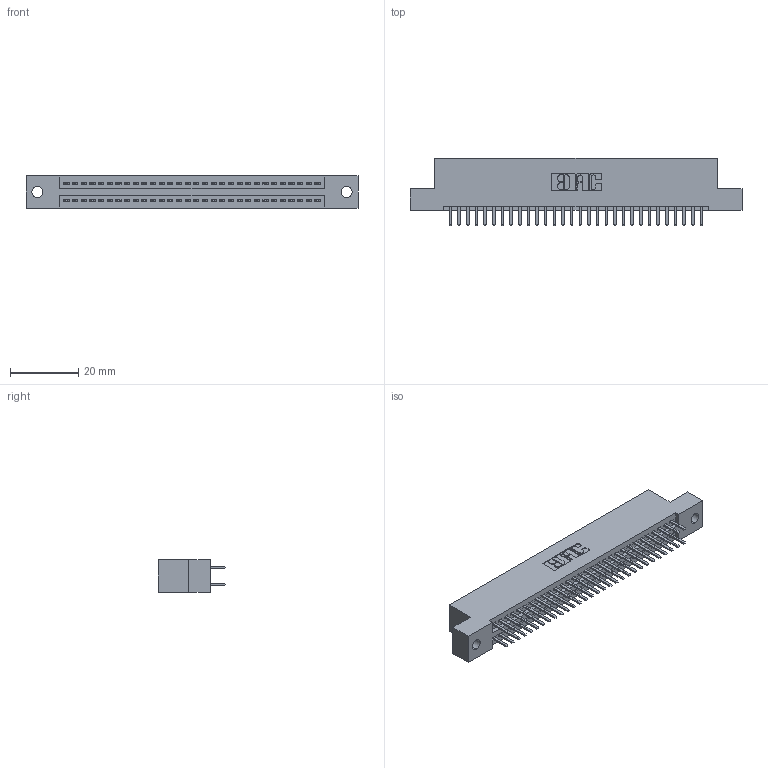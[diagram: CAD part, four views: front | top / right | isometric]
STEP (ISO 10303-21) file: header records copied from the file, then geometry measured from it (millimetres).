
FILE_DESCRIPTION (( 'STEP AP203' ), '1' );
FILE_NAME ('395-060-520-202.STEP', '2018-11-23T10:31:42', ( '' ), ( '' ), 'SwSTEP 2.0', 'SolidWorks 2016', '' );
FILE_SCHEMA (( 'CONFIG_CONTROL_DESIGN' ));
Length unit declared in the file: inch
Products named in the file (3): 345-292-001_345-293-120; 345 Part_Flush Mounting Lugs - 0.128 Dia; 395-060-520-202
Assembly tree (61 placements, depth 2):
  395-060-520-202
    345 Part_Flush Mounting Lugs - 0.128 Dia
    345-292-001_345-293-120  x60
Bounding box: 97.41 x 19.68 x 9.4 mm (x, y, z)
Volume: 9288 mm3; surface area: 13167.9 mm2
Topology: 61 solids, 61 shells, 3366 faces, 9761 edges, 6346 vertices
Faces by surface type: plane 2180, cylinder 1186
Entity records: 25271 total; most frequent: CARTESIAN_POINT 4260, ORIENTED_EDGE 4182, DIRECTION 3759, EDGE_CURVE 2091, LINE 1835, VECTOR 1835, VERTEX_POINT 1390, AXIS2_PLACEMENT_3D 962
